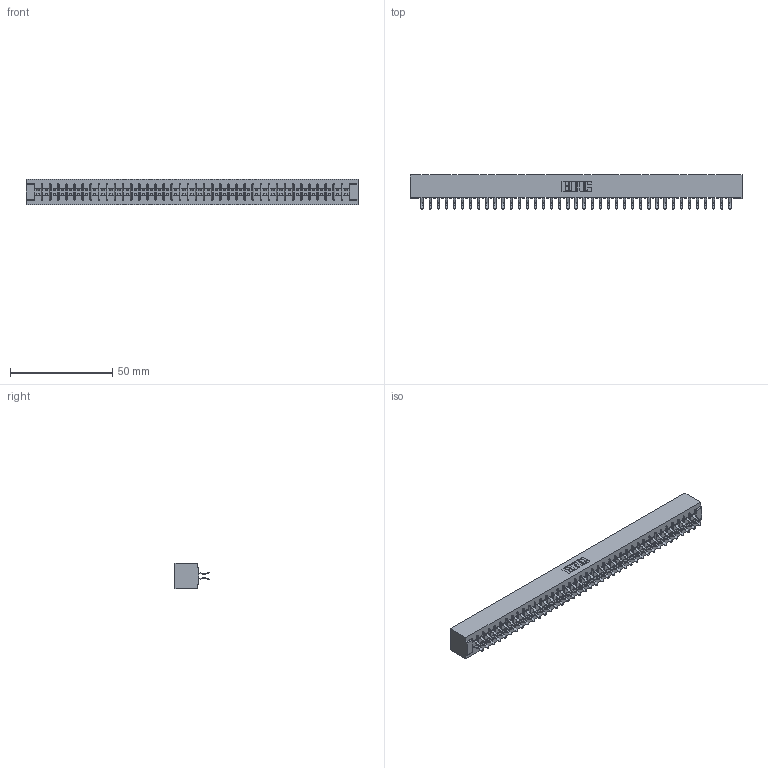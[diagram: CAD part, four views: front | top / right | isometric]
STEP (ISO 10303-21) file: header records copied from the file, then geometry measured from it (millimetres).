
FILE_DESCRIPTION (( 'STEP AP203' ), '1' );
FILE_NAME ('355-078-556-201.STEP', '2019-09-13T14:08:21', ( '' ), ( '' ), 'SwSTEP 2.0', 'SolidWorks 2016', '' );
FILE_SCHEMA (( 'CONFIG_CONTROL_DESIGN' ));
Length unit declared in the file: inch
Products named in the file (3): 355-078-556-201; 305-290-001_556; 305 Part_No Mounting
Assembly tree (79 placements, depth 2):
  355-078-556-201
    305 Part_No Mounting
    305-290-001_556  x78
Bounding box: 162.41 x 16.64 x 12.7 mm (x, y, z)
Volume: 17391.9 mm3; surface area: 22501.8 mm2
Topology: 79 solids, 79 shells, 4476 faces, 12889 edges, 8382 vertices
Faces by surface type: plane 2482, cylinder 1838, sphere 156
Entity records: 42536 total; most frequent: CARTESIAN_POINT 7039, ORIENTED_EDGE 6986, DIRECTION 6813, EDGE_CURVE 3493, VECTOR 2821, LINE 2821, VERTEX_POINT 2222, AXIS2_PLACEMENT_3D 1996
